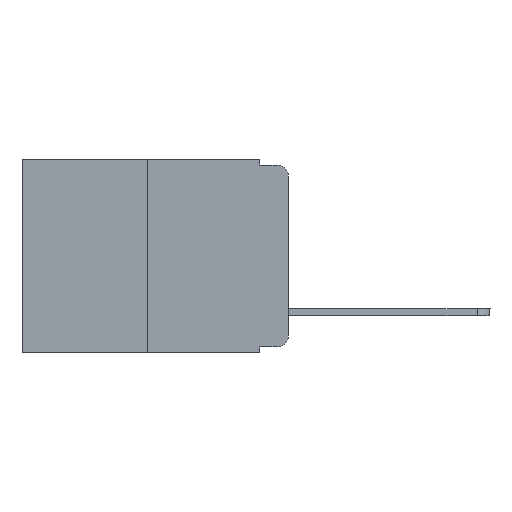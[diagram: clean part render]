
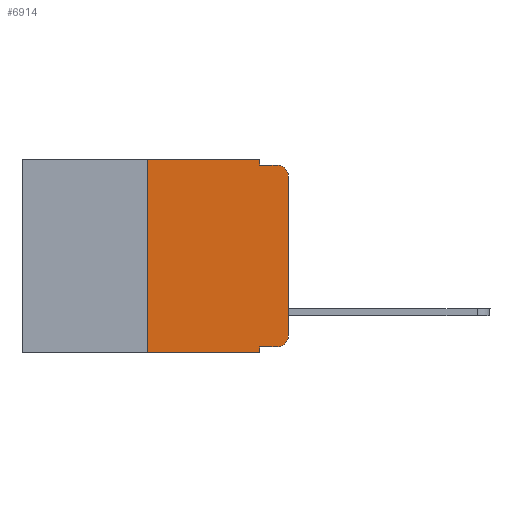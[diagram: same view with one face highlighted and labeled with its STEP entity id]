
A CAD part, left-side view. The second image highlights one B-rep face of the part: STEP entity #6914.
In plain terms, the highlighted planar face has unit normal (-1, 0, 0).
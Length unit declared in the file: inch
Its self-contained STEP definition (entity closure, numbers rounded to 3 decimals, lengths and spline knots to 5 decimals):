
#355 = AXIS2_PLACEMENT_3D ( 'NONE', #12703, #20198, #14538 ) ;
#661 = ORIENTED_EDGE ( 'NONE', *, *, #14910, .T. ) ;
#1070 = EDGE_CURVE ( 'NONE', #12438, #11838, #18294, .T. ) ;
#1576 = CARTESIAN_POINT ( 'NONE',  ( 0., 0.02, -0.333 ) ) ;
#1591 = VECTOR ( 'NONE', #5191, 39.37008 ) ;
#1634 = VECTOR ( 'NONE', #6701, 39.37008 ) ;
#1719 = VECTOR ( 'NONE', #14385, 39.37008 ) ;
#1727 = EDGE_CURVE ( 'NONE', #12019, #2859, #17266, .T. ) ;
#2859 = VERTEX_POINT ( 'NONE', #19332 ) ;
#3282 = ORIENTED_EDGE ( 'NONE', *, *, #1727, .T. ) ;
#3308 = VECTOR ( 'NONE', #5595, 39.37008 ) ;
#3555 = LINE ( 'NONE', #14686, #22820 ) ;
#3647 = DIRECTION ( 'NONE',  ( 0., 0., -1. ) ) ;
#3885 = ORIENTED_EDGE ( 'NONE', *, *, #13162, .F. ) ;
#4010 = CARTESIAN_POINT ( 'NONE',  ( 0., 0.051, 0. ) ) ;
#4037 = CARTESIAN_POINT ( 'NONE',  ( 0., 0.02, -0.03 ) ) ;
#4185 = CARTESIAN_POINT ( 'NONE',  ( 0., 0.473, 0. ) ) ;
#4899 = VERTEX_POINT ( 'NONE', #7131 ) ;
#5042 = ORIENTED_EDGE ( 'NONE', *, *, #19732, .T. ) ;
#5191 = DIRECTION ( 'NONE',  ( 0., -1., 0. ) ) ;
#5463 = CARTESIAN_POINT ( 'NONE',  ( 0., 0.051, -0.333 ) ) ;
#5595 = DIRECTION ( 'NONE',  ( 0., 0., -1. ) ) ;
#5884 = PLANE ( 'NONE',  #22239 ) ;
#6619 = CIRCLE ( 'NONE', #9729, 0.02 ) ;
#6701 = DIRECTION ( 'NONE',  ( 0., -1., 0. ) ) ;
#6914 = ADVANCED_FACE ( 'NONE', ( #16910 ), #5884, .F. ) ;
#6959 = CIRCLE ( 'NONE', #355, 0.02 ) ;
#7021 = CARTESIAN_POINT ( 'NONE',  ( 0., 0.25, 0. ) ) ;
#7131 = CARTESIAN_POINT ( 'NONE',  ( 0., 0., -0.03 ) ) ;
#7458 = ORIENTED_EDGE ( 'NONE', *, *, #1070, .F. ) ;
#7821 = DIRECTION ( 'NONE',  ( 1., 0., 0. ) ) ;
#7881 = VERTEX_POINT ( 'NONE', #7021 ) ;
#8053 = CARTESIAN_POINT ( 'NONE',  ( 0., 0.25, 0. ) ) ;
#8319 = VERTEX_POINT ( 'NONE', #16292 ) ;
#8781 = ORIENTED_EDGE ( 'NONE', *, *, #21132, .F. ) ;
#8975 = VECTOR ( 'NONE', #22680, 39.37008 ) ;
#9228 = DIRECTION ( 'NONE',  ( 0., 0., 1. ) ) ;
#9352 = CARTESIAN_POINT ( 'NONE',  ( 0., 0.25, -0.343 ) ) ;
#9729 = AXIS2_PLACEMENT_3D ( 'NONE', #4037, #15177, #20703 ) ;
#10417 = CARTESIAN_POINT ( 'NONE',  ( 0., 0.02, -0.01 ) ) ;
#10502 = CARTESIAN_POINT ( 'NONE',  ( 0., 0.051, -0.01 ) ) ;
#11001 = ORIENTED_EDGE ( 'NONE', *, *, #23438, .F. ) ;
#11838 = VERTEX_POINT ( 'NONE', #18190 ) ;
#12019 = VERTEX_POINT ( 'NONE', #9352 ) ;
#12269 = VERTEX_POINT ( 'NONE', #10417 ) ;
#12287 = ORIENTED_EDGE ( 'NONE', *, *, #13528, .F. ) ;
#12416 = VERTEX_POINT ( 'NONE', #5463 ) ;
#12438 = VERTEX_POINT ( 'NONE', #16604 ) ;
#12703 = CARTESIAN_POINT ( 'NONE',  ( 0., 0.02, -0.313 ) ) ;
#12867 = VECTOR ( 'NONE', #20872, 39.37008 ) ;
#13062 = ORIENTED_EDGE ( 'NONE', *, *, #18734, .T. ) ;
#13162 = EDGE_CURVE ( 'NONE', #12416, #2859, #18647, .T. ) ;
#13183 = VERTEX_POINT ( 'NONE', #1576 ) ;
#13528 = EDGE_CURVE ( 'NONE', #7881, #12438, #21978, .T. ) ;
#13910 = EDGE_CURVE ( 'NONE', #4899, #12269, #6619, .T. ) ;
#14385 = DIRECTION ( 'NONE',  ( 0., -1., 0. ) ) ;
#14501 = LINE ( 'NONE', #10502, #1719 ) ;
#14538 = DIRECTION ( 'NONE',  ( 0., 0., -1. ) ) ;
#14686 = CARTESIAN_POINT ( 'NONE',  ( 0., 0., 0. ) ) ;
#14910 = EDGE_CURVE ( 'NONE', #12416, #13183, #20989, .T. ) ;
#15177 = DIRECTION ( 'NONE',  ( -1., 0., 0. ) ) ;
#15200 = DIRECTION ( 'NONE',  ( 0., 0., -1. ) ) ;
#15236 = CARTESIAN_POINT ( 'NONE',  ( 0., 0.051, -0.333 ) ) ;
#15717 = ORIENTED_EDGE ( 'NONE', *, *, #13910, .T. ) ;
#16292 = CARTESIAN_POINT ( 'NONE',  ( 0., 0., -0.313 ) ) ;
#16604 = CARTESIAN_POINT ( 'NONE',  ( 0., 0.051, 0. ) ) ;
#16910 = FACE_OUTER_BOUND ( 'NONE', #18107, .T. ) ;
#17266 = LINE ( 'NONE', #23269, #1634 ) ;
#18107 = EDGE_LOOP ( 'NONE', ( #5042, #15717, #11001, #7458, #12287, #8781, #3282, #3885, #661, #13062 ) ) ;
#18190 = CARTESIAN_POINT ( 'NONE',  ( 0., 0.051, -0.01 ) ) ;
#18294 = LINE ( 'NONE', #4010, #3308 ) ;
#18647 = LINE ( 'NONE', #22369, #20499 ) ;
#18734 = EDGE_CURVE ( 'NONE', #13183, #8319, #6959, .T. ) ;
#19332 = CARTESIAN_POINT ( 'NONE',  ( 0., 0.051, -0.343 ) ) ;
#19732 = EDGE_CURVE ( 'NONE', #8319, #4899, #3555, .T. ) ;
#20050 = CARTESIAN_POINT ( 'NONE',  ( 0., 0.473, 0. ) ) ;
#20198 = DIRECTION ( 'NONE',  ( -1., 0., 0. ) ) ;
#20499 = VECTOR ( 'NONE', #3647, 39.37008 ) ;
#20703 = DIRECTION ( 'NONE',  ( 0., 0., -1. ) ) ;
#20839 = LINE ( 'NONE', #8053, #8975 ) ;
#20872 = DIRECTION ( 'NONE',  ( 0., -1., 0. ) ) ;
#20989 = LINE ( 'NONE', #15236, #12867 ) ;
#21132 = EDGE_CURVE ( 'NONE', #12019, #7881, #20839, .T. ) ;
#21978 = LINE ( 'NONE', #20050, #1591 ) ;
#22239 = AXIS2_PLACEMENT_3D ( 'NONE', #4185, #7821, #15200 ) ;
#22369 = CARTESIAN_POINT ( 'NONE',  ( 0., 0.051, 0. ) ) ;
#22680 = DIRECTION ( 'NONE',  ( 0., 0., 1. ) ) ;
#22820 = VECTOR ( 'NONE', #9228, 39.37008 ) ;
#23269 = CARTESIAN_POINT ( 'NONE',  ( 0., 0.473, -0.343 ) ) ;
#23438 = EDGE_CURVE ( 'NONE', #11838, #12269, #14501, .T. ) ;
